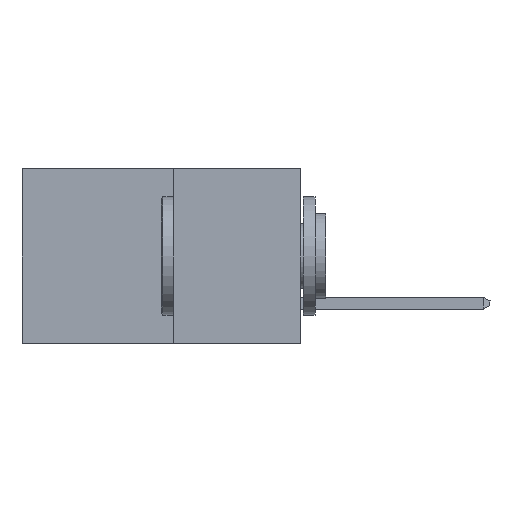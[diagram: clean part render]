
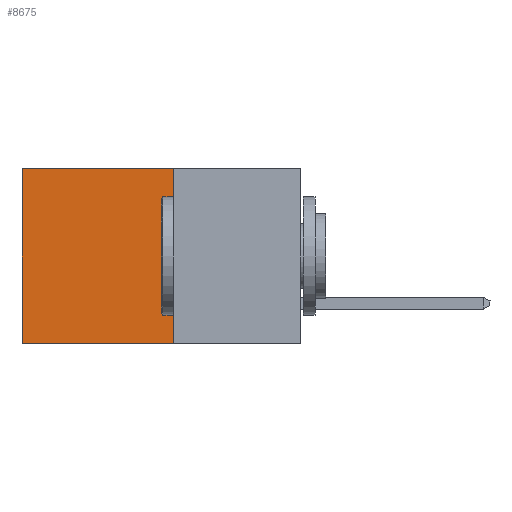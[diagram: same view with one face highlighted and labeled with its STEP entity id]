
A CAD part, left-side view. The second image highlights one B-rep face of the part: STEP entity #8675.
In plain terms, the highlighted planar face has unit normal (-1, 0, 0).
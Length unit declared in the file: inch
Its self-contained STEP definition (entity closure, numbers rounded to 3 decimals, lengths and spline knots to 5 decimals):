
#182 = VERTEX_POINT ( 'NONE', #4194 ) ;
#1598 = EDGE_CURVE ( 'NONE', #6558, #8508, #6022, .T. ) ;
#1884 = CARTESIAN_POINT ( 'NONE',  ( 0.277, 0.27, -0.37 ) ) ;
#1931 = LINE ( 'NONE', #11360, #12323 ) ;
#2207 = VECTOR ( 'NONE', #10547, 39.37008 ) ;
#2701 = DIRECTION ( 'NONE',  ( 0., 1., 0. ) ) ;
#2744 = CARTESIAN_POINT ( 'NONE',  ( 0.277, 0.27, 0. ) ) ;
#2957 = ORIENTED_EDGE ( 'NONE', *, *, #3253, .F. ) ;
#3087 = EDGE_CURVE ( 'NONE', #182, #6558, #6391, .T. ) ;
#3127 = AXIS2_PLACEMENT_3D ( 'NONE', #7945, #7275, #7269 ) ;
#3253 = EDGE_CURVE ( 'NONE', #5396, #8508, #1931, .T. ) ;
#3518 = VECTOR ( 'NONE', #2701, 39.37008 ) ;
#3823 = ORIENTED_EDGE ( 'NONE', *, *, #3087, .T. ) ;
#4194 = CARTESIAN_POINT ( 'NONE',  ( 0.277, 0.27, 0. ) ) ;
#4412 = FACE_OUTER_BOUND ( 'NONE', #12310, .T. ) ;
#5396 = VERTEX_POINT ( 'NONE', #1884 ) ;
#6022 = LINE ( 'NONE', #6283, #11268 ) ;
#6270 = DIRECTION ( 'NONE',  ( 0., 0., -1. ) ) ;
#6283 = CARTESIAN_POINT ( 'NONE',  ( 0.277, 0.59, -0.37 ) ) ;
#6391 = LINE ( 'NONE', #2744, #3518 ) ;
#6558 = VERTEX_POINT ( 'NONE', #6694 ) ;
#6694 = CARTESIAN_POINT ( 'NONE',  ( 0.277, 0.59, 0. ) ) ;
#7269 = DIRECTION ( 'NONE',  ( 0., 0., -1. ) ) ;
#7275 = DIRECTION ( 'NONE',  ( 1., 0., 0. ) ) ;
#7302 = PLANE ( 'NONE',  #3127 ) ;
#7945 = CARTESIAN_POINT ( 'NONE',  ( 0.277, 0.27, -0.37 ) ) ;
#8500 = ORIENTED_EDGE ( 'NONE', *, *, #1598, .T. ) ;
#8508 = VERTEX_POINT ( 'NONE', #9515 ) ;
#8675 = ADVANCED_FACE ( 'NONE', ( #4412 ), #7302, .F. ) ;
#8874 = EDGE_CURVE ( 'NONE', #182, #5396, #9900, .T. ) ;
#9515 = CARTESIAN_POINT ( 'NONE',  ( 0.277, 0.59, -0.37 ) ) ;
#9900 = LINE ( 'NONE', #11035, #2207 ) ;
#10547 = DIRECTION ( 'NONE',  ( 0., 0., -1. ) ) ;
#11035 = CARTESIAN_POINT ( 'NONE',  ( 0.277, 0.27, -0.37 ) ) ;
#11268 = VECTOR ( 'NONE', #6270, 39.37008 ) ;
#11360 = CARTESIAN_POINT ( 'NONE',  ( 0.277, 0.27, -0.37 ) ) ;
#11376 = DIRECTION ( 'NONE',  ( 0., 1., 0. ) ) ;
#12310 = EDGE_LOOP ( 'NONE', ( #8500, #2957, #12605, #3823 ) ) ;
#12323 = VECTOR ( 'NONE', #11376, 39.37008 ) ;
#12605 = ORIENTED_EDGE ( 'NONE', *, *, #8874, .F. ) ;
